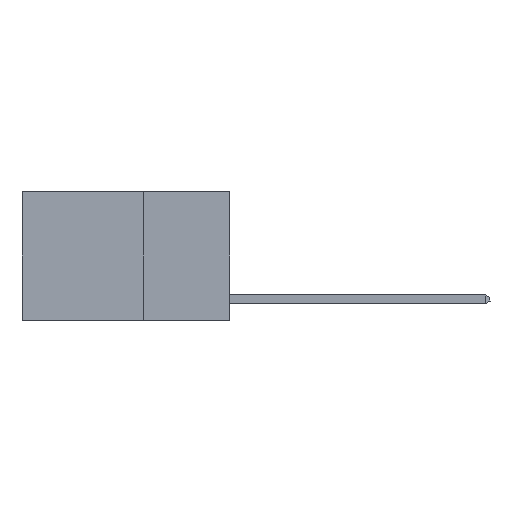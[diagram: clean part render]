
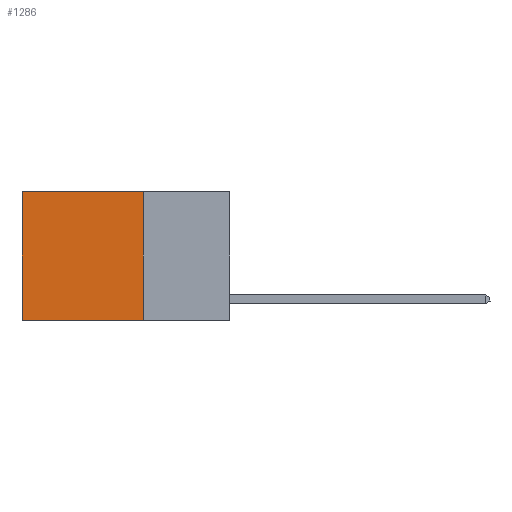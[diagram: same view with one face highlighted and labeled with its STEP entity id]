
A CAD part, left-side view. The second image highlights one B-rep face of the part: STEP entity #1286.
In plain terms, the highlighted planar face has unit normal (-1, 0, 0).
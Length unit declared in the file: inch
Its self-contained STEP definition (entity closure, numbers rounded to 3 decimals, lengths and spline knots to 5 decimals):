
#881 = LINE ( 'NONE', #25446, #23721 ) ;
#1286 = ADVANCED_FACE ( 'NONE', ( #8236 ), #27083, .F. ) ;
#2617 = CARTESIAN_POINT ( 'NONE',  ( 0.2625, 0.25, -0.37 ) ) ;
#2817 = DIRECTION ( 'NONE',  ( 0., 1., 0. ) ) ;
#2981 = VERTEX_POINT ( 'NONE', #4422 ) ;
#3644 = LINE ( 'NONE', #17169, #7268 ) ;
#3884 = ORIENTED_EDGE ( 'NONE', *, *, #6351, .F. ) ;
#4174 = DIRECTION ( 'NONE',  ( 1., 0., 0. ) ) ;
#4422 = CARTESIAN_POINT ( 'NONE',  ( 0.2625, 0.6, 0. ) ) ;
#4644 = EDGE_CURVE ( 'NONE', #8563, #2981, #881, .T. ) ;
#5282 = EDGE_LOOP ( 'NONE', ( #23737, #3884, #22424, #12103 ) ) ;
#5626 = DIRECTION ( 'NONE',  ( 0., 0., -1. ) ) ;
#6351 = EDGE_CURVE ( 'NONE', #8860, #11479, #25096, .T. ) ;
#6580 = CARTESIAN_POINT ( 'NONE',  ( 0.2625, 0.6, -0.37 ) ) ;
#7268 = VECTOR ( 'NONE', #15534, 39.37008 ) ;
#8236 = FACE_OUTER_BOUND ( 'NONE', #5282, .T. ) ;
#8563 = VERTEX_POINT ( 'NONE', #29846 ) ;
#8860 = VERTEX_POINT ( 'NONE', #12604 ) ;
#10678 = CARTESIAN_POINT ( 'NONE',  ( 0.2625, 0.25, 0. ) ) ;
#11479 = VERTEX_POINT ( 'NONE', #6580 ) ;
#11784 = LINE ( 'NONE', #17405, #21229 ) ;
#12103 = ORIENTED_EDGE ( 'NONE', *, *, #4644, .T. ) ;
#12604 = CARTESIAN_POINT ( 'NONE',  ( 0.2625, 0.25, -0.37 ) ) ;
#12765 = VECTOR ( 'NONE', #2817, 39.37008 ) ;
#14224 = EDGE_CURVE ( 'NONE', #2981, #11479, #3644, .T. ) ;
#15534 = DIRECTION ( 'NONE',  ( 0., 0., -1. ) ) ;
#15776 = DIRECTION ( 'NONE',  ( 0., 0., -1. ) ) ;
#17169 = CARTESIAN_POINT ( 'NONE',  ( 0.2625, 0.6, 0. ) ) ;
#17222 = EDGE_CURVE ( 'NONE', #8563, #8860, #11784, .T. ) ;
#17405 = CARTESIAN_POINT ( 'NONE',  ( 0.2625, 0.25, 0. ) ) ;
#19888 = AXIS2_PLACEMENT_3D ( 'NONE', #10678, #4174, #15776 ) ;
#21229 = VECTOR ( 'NONE', #5626, 39.37008 ) ;
#22424 = ORIENTED_EDGE ( 'NONE', *, *, #17222, .F. ) ;
#23721 = VECTOR ( 'NONE', #29770, 39.37008 ) ;
#23737 = ORIENTED_EDGE ( 'NONE', *, *, #14224, .T. ) ;
#25096 = LINE ( 'NONE', #2617, #12765 ) ;
#25446 = CARTESIAN_POINT ( 'NONE',  ( 0.2625, 0.25, 0. ) ) ;
#27083 = PLANE ( 'NONE',  #19888 ) ;
#29770 = DIRECTION ( 'NONE',  ( 0., 1., 0. ) ) ;
#29846 = CARTESIAN_POINT ( 'NONE',  ( 0.2625, 0.25, 0. ) ) ;
